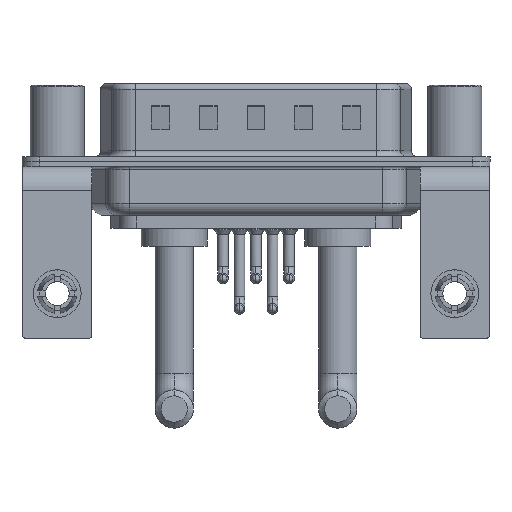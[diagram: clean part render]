
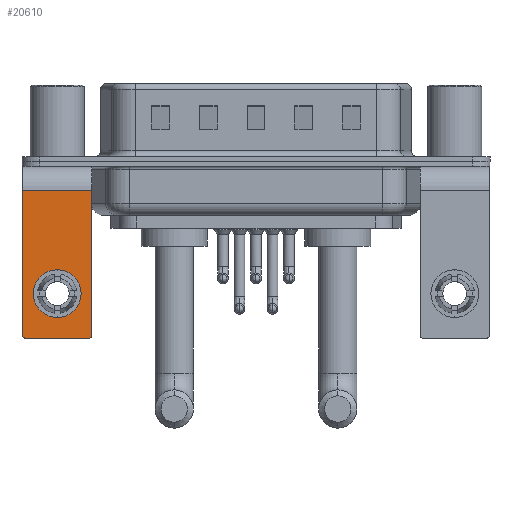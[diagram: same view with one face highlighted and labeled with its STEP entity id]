
A CAD part, front view. The second image highlights one B-rep face of the part: STEP entity #20610.
In plain terms, the highlighted planar face has unit normal (0, -1, 0).
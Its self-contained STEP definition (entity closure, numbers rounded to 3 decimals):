
#152 = CIRCLE ( 'NONE', #4489, 0.25 ) ;
#170 = CARTESIAN_POINT ( 'NONE',  ( 0., -6.25, -9.07 ) ) ;
#325 = EDGE_CURVE ( 'NONE', #1533, #5336, #24407, .T. ) ;
#646 = ORIENTED_EDGE ( 'NONE', *, *, #17152, .F. ) ;
#1411 = AXIS2_PLACEMENT_3D ( 'NONE', #15961, #3180, #23509 ) ;
#1509 = AXIS2_PLACEMENT_3D ( 'NONE', #19495, #23174, #13761 ) ;
#1524 = ORIENTED_EDGE ( 'NONE', *, *, #11966, .T. ) ;
#1533 = VERTEX_POINT ( 'NONE', #16900 ) ;
#2015 = EDGE_CURVE ( 'NONE', #24475, #13378, #152, .T. ) ;
#2588 = CIRCLE ( 'NONE', #1411, 2. ) ;
#3119 = CIRCLE ( 'NONE', #21336, 0.25 ) ;
#3180 = DIRECTION ( 'NONE',  ( 0., 1., 0. ) ) ;
#3184 = EDGE_CURVE ( 'NONE', #11814, #1533, #5129, .T. ) ;
#3245 = CARTESIAN_POINT ( 'NONE',  ( 2.65, -6.25, -14.55 ) ) ;
#3720 = CARTESIAN_POINT ( 'NONE',  ( -2.9, -6.25, -2.4 ) ) ;
#4443 = EDGE_CURVE ( 'NONE', #23799, #8876, #2588, .T. ) ;
#4489 = AXIS2_PLACEMENT_3D ( 'NONE', #3245, #14663, #22902 ) ;
#4930 = LINE ( 'NONE', #14117, #19792 ) ;
#5129 = LINE ( 'NONE', #18157, #15207 ) ;
#5336 = VERTEX_POINT ( 'NONE', #19666 ) ;
#5505 = ORIENTED_EDGE ( 'NONE', *, *, #325, .T. ) ;
#5594 = CARTESIAN_POINT ( 'NONE',  ( 2.9, -6.25, -2.4 ) ) ;
#5770 = CARTESIAN_POINT ( 'NONE',  ( 2.9, -6.25, -2.4 ) ) ;
#6141 = DIRECTION ( 'NONE',  ( 0., 0., 1. ) ) ;
#6799 = DIRECTION ( 'NONE',  ( 0., 0., -1. ) ) ;
#7561 = CARTESIAN_POINT ( 'NONE',  ( -2.65, -6.25, -14.8 ) ) ;
#7639 = FACE_BOUND ( 'NONE', #20354, .T. ) ;
#7706 = DIRECTION ( 'NONE',  ( 0., -1., 0. ) ) ;
#8655 = CARTESIAN_POINT ( 'NONE',  ( 2.9, -6.25, -14.8 ) ) ;
#8876 = VERTEX_POINT ( 'NONE', #11986 ) ;
#9468 = VECTOR ( 'NONE', #19708, 1000. ) ;
#9505 = FACE_OUTER_BOUND ( 'NONE', #14836, .T. ) ;
#9788 = DIRECTION ( 'NONE',  ( 0., 0., -1. ) ) ;
#10526 = ORIENTED_EDGE ( 'NONE', *, *, #4443, .T. ) ;
#11014 = ORIENTED_EDGE ( 'NONE', *, *, #17218, .F. ) ;
#11814 = VERTEX_POINT ( 'NONE', #5594 ) ;
#11966 = EDGE_CURVE ( 'NONE', #8876, #23799, #20119, .T. ) ;
#11986 = CARTESIAN_POINT ( 'NONE',  ( 0., -6.25, -13.07 ) ) ;
#12698 = DIRECTION ( 'NONE',  ( -1., 0., 0. ) ) ;
#13378 = VERTEX_POINT ( 'NONE', #23917 ) ;
#13545 = VERTEX_POINT ( 'NONE', #7561 ) ;
#13549 = VECTOR ( 'NONE', #9788, 1000. ) ;
#13761 = DIRECTION ( 'NONE',  ( 0., 0., 1. ) ) ;
#14117 = CARTESIAN_POINT ( 'NONE',  ( 2.9, -6.25, -2.4 ) ) ;
#14257 = ORIENTED_EDGE ( 'NONE', *, *, #14843, .T. ) ;
#14663 = DIRECTION ( 'NONE',  ( 0., -1., 0. ) ) ;
#14836 = EDGE_LOOP ( 'NONE', ( #5505, #14257, #11014, #14915, #646, #20844 ) ) ;
#14843 = EDGE_CURVE ( 'NONE', #5336, #13545, #3119, .T. ) ;
#14915 = ORIENTED_EDGE ( 'NONE', *, *, #2015, .T. ) ;
#15207 = VECTOR ( 'NONE', #12698, 1000. ) ;
#15961 = CARTESIAN_POINT ( 'NONE',  ( 0., -6.25, -11.07 ) ) ;
#16455 = CARTESIAN_POINT ( 'NONE',  ( 2.65, -6.25, -14.8 ) ) ;
#16900 = CARTESIAN_POINT ( 'NONE',  ( -2.9, -6.25, -2.4 ) ) ;
#16938 = DIRECTION ( 'NONE',  ( 0., 1., 0. ) ) ;
#17137 = CARTESIAN_POINT ( 'NONE',  ( -2.65, -6.25, -14.55 ) ) ;
#17152 = EDGE_CURVE ( 'NONE', #11814, #13378, #4930, .T. ) ;
#17218 = EDGE_CURVE ( 'NONE', #24475, #13545, #23783, .T. ) ;
#17308 = PLANE ( 'NONE',  #18936 ) ;
#18157 = CARTESIAN_POINT ( 'NONE',  ( 2.9, -6.25, -2.4 ) ) ;
#18936 = AXIS2_PLACEMENT_3D ( 'NONE', #5770, #16938, #6141 ) ;
#19495 = CARTESIAN_POINT ( 'NONE',  ( 0., -6.25, -11.07 ) ) ;
#19666 = CARTESIAN_POINT ( 'NONE',  ( -2.9, -6.25, -14.55 ) ) ;
#19708 = DIRECTION ( 'NONE',  ( -1., 0., 0. ) ) ;
#19792 = VECTOR ( 'NONE', #6799, 1000. ) ;
#20119 = CIRCLE ( 'NONE', #1509, 2. ) ;
#20354 = EDGE_LOOP ( 'NONE', ( #1524, #10526 ) ) ;
#20610 = ADVANCED_FACE ( 'NONE', ( #7639, #9505 ), #17308, .F. ) ;
#20844 = ORIENTED_EDGE ( 'NONE', *, *, #3184, .T. ) ;
#21336 = AXIS2_PLACEMENT_3D ( 'NONE', #17137, #7706, #22696 ) ;
#22696 = DIRECTION ( 'NONE',  ( 0., 0., 1. ) ) ;
#22902 = DIRECTION ( 'NONE',  ( 0., 0., 1. ) ) ;
#23174 = DIRECTION ( 'NONE',  ( 0., 1., 0. ) ) ;
#23509 = DIRECTION ( 'NONE',  ( 0., 0., 1. ) ) ;
#23783 = LINE ( 'NONE', #8655, #9468 ) ;
#23799 = VERTEX_POINT ( 'NONE', #170 ) ;
#23917 = CARTESIAN_POINT ( 'NONE',  ( 2.9, -6.25, -14.55 ) ) ;
#24407 = LINE ( 'NONE', #3720, #13549 ) ;
#24475 = VERTEX_POINT ( 'NONE', #16455 ) ;
